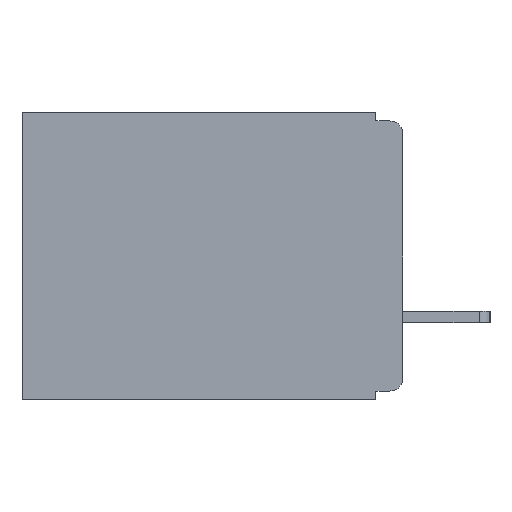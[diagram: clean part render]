
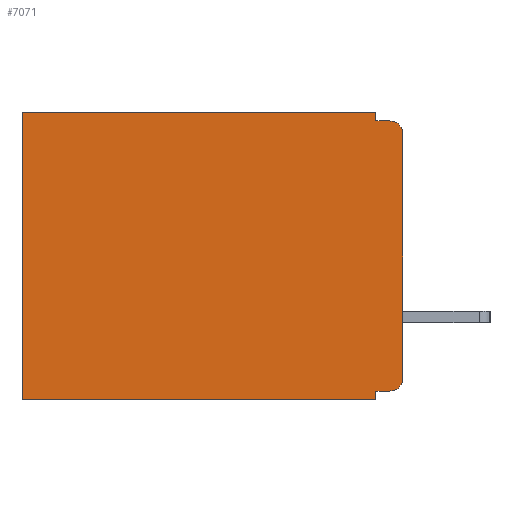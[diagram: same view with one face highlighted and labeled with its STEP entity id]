
A CAD part, left-side view. The second image highlights one B-rep face of the part: STEP entity #7071.
In plain terms, the highlighted planar face has unit normal (-1, 0, 0).
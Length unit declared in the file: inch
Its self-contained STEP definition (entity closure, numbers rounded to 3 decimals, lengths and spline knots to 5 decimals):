
#263 = DIRECTION ( 'NONE',  ( 0., 0., -1. ) ) ;
#1427 = EDGE_CURVE ( 'NONE', #22461, #13927, #12669, .T. ) ;
#1636 = CARTESIAN_POINT ( 'NONE',  ( 0.3, 0., -0.305 ) ) ;
#1752 = CARTESIAN_POINT ( 'NONE',  ( 0.3, 0., -0.01 ) ) ;
#1846 = CIRCLE ( 'NONE', #20642, 0.015 ) ;
#2323 = EDGE_CURVE ( 'NONE', #16897, #26285, #1846, .T. ) ;
#2445 = PLANE ( 'NONE',  #14420 ) ;
#2568 = LINE ( 'NONE', #6167, #17418 ) ;
#2995 = CARTESIAN_POINT ( 'NONE',  ( 0.3, 0.031, 0. ) ) ;
#4629 = CARTESIAN_POINT ( 'NONE',  ( 0.3, 0.031, -0.33 ) ) ;
#4655 = DIRECTION ( 'NONE',  ( 1., 0., 0. ) ) ;
#4882 = ORIENTED_EDGE ( 'NONE', *, *, #13076, .F. ) ;
#5349 = DIRECTION ( 'NONE',  ( 0., -1., 0. ) ) ;
#5453 = CARTESIAN_POINT ( 'NONE',  ( 0.3, 0.437, 0. ) ) ;
#5562 = ORIENTED_EDGE ( 'NONE', *, *, #15362, .F. ) ;
#5638 = ORIENTED_EDGE ( 'NONE', *, *, #25795, .F. ) ;
#5671 = EDGE_CURVE ( 'NONE', #23626, #6668, #13593, .T. ) ;
#5767 = VERTEX_POINT ( 'NONE', #4629 ) ;
#5918 = EDGE_CURVE ( 'NONE', #24119, #22461, #17615, .T. ) ;
#6129 = ORIENTED_EDGE ( 'NONE', *, *, #2323, .T. ) ;
#6167 = CARTESIAN_POINT ( 'NONE',  ( 0.3, 0., 0. ) ) ;
#6527 = LINE ( 'NONE', #26461, #23247 ) ;
#6556 = ORIENTED_EDGE ( 'NONE', *, *, #19718, .F. ) ;
#6668 = VERTEX_POINT ( 'NONE', #25015 ) ;
#7071 = ADVANCED_FACE ( 'NONE', ( #24930 ), #2445, .F. ) ;
#7114 = CIRCLE ( 'NONE', #18214, 0.015 ) ;
#9069 = DIRECTION ( 'NONE',  ( -1., 0., 0. ) ) ;
#9681 = ORIENTED_EDGE ( 'NONE', *, *, #21355, .T. ) ;
#10039 = VERTEX_POINT ( 'NONE', #13477 ) ;
#10430 = CARTESIAN_POINT ( 'NONE',  ( 0.3, 0., -0.32 ) ) ;
#10809 = VECTOR ( 'NONE', #22095, 39.37008 ) ;
#11043 = CARTESIAN_POINT ( 'NONE',  ( 0.3, 0., -0.33 ) ) ;
#11328 = CARTESIAN_POINT ( 'NONE',  ( 0.3, 0., -0.33 ) ) ;
#11842 = VECTOR ( 'NONE', #20567, 39.37008 ) ;
#11960 = VECTOR ( 'NONE', #5349, 39.37008 ) ;
#12669 = LINE ( 'NONE', #1752, #11960 ) ;
#13076 = EDGE_CURVE ( 'NONE', #10039, #5767, #15922, .T. ) ;
#13277 = DIRECTION ( 'NONE',  ( 0., 1., 0. ) ) ;
#13327 = VERTEX_POINT ( 'NONE', #18680 ) ;
#13381 = CARTESIAN_POINT ( 'NONE',  ( 0.3, 0.031, -0.01 ) ) ;
#13477 = CARTESIAN_POINT ( 'NONE',  ( 0.3, 0.031, -0.32 ) ) ;
#13593 = LINE ( 'NONE', #15315, #25007 ) ;
#13927 = VERTEX_POINT ( 'NONE', #18648 ) ;
#14420 = AXIS2_PLACEMENT_3D ( 'NONE', #11328, #4655, #20041 ) ;
#14569 = LINE ( 'NONE', #11043, #20295 ) ;
#14839 = DIRECTION ( 'NONE',  ( 0., 1., 0. ) ) ;
#15315 = CARTESIAN_POINT ( 'NONE',  ( 0.3, 0.437, -0.33 ) ) ;
#15362 = EDGE_CURVE ( 'NONE', #16897, #10039, #17183, .T. ) ;
#15366 = ORIENTED_EDGE ( 'NONE', *, *, #21829, .T. ) ;
#15611 = CARTESIAN_POINT ( 'NONE',  ( 0.3, 0.031, -0.33 ) ) ;
#15922 = LINE ( 'NONE', #15611, #10809 ) ;
#16897 = VERTEX_POINT ( 'NONE', #22459 ) ;
#17170 = EDGE_LOOP ( 'NONE', ( #6556, #9681, #21881, #23329, #15366, #23208, #5638, #4882, #5562, #6129 ) ) ;
#17183 = LINE ( 'NONE', #10430, #27898 ) ;
#17418 = VECTOR ( 'NONE', #25778, 39.37008 ) ;
#17615 = LINE ( 'NONE', #2995, #11842 ) ;
#18214 = AXIS2_PLACEMENT_3D ( 'NONE', #22086, #9069, #24244 ) ;
#18648 = CARTESIAN_POINT ( 'NONE',  ( 0.3, 0.015, -0.01 ) ) ;
#18680 = CARTESIAN_POINT ( 'NONE',  ( 0.3, 0., -0.025 ) ) ;
#19718 = EDGE_CURVE ( 'NONE', #13327, #26285, #6527, .T. ) ;
#20041 = DIRECTION ( 'NONE',  ( 0., 0., -1. ) ) ;
#20295 = VECTOR ( 'NONE', #13277, 39.37008 ) ;
#20567 = DIRECTION ( 'NONE',  ( 0., 0., -1. ) ) ;
#20580 = DIRECTION ( 'NONE',  ( -1., 0., 0. ) ) ;
#20642 = AXIS2_PLACEMENT_3D ( 'NONE', #26998, #20580, #23226 ) ;
#21355 = EDGE_CURVE ( 'NONE', #13327, #13927, #7114, .T. ) ;
#21829 = EDGE_CURVE ( 'NONE', #24119, #23626, #2568, .T. ) ;
#21881 = ORIENTED_EDGE ( 'NONE', *, *, #1427, .F. ) ;
#22086 = CARTESIAN_POINT ( 'NONE',  ( 0.3, 0.015, -0.025 ) ) ;
#22095 = DIRECTION ( 'NONE',  ( 0., 0., -1. ) ) ;
#22459 = CARTESIAN_POINT ( 'NONE',  ( 0.3, 0.015, -0.32 ) ) ;
#22461 = VERTEX_POINT ( 'NONE', #13381 ) ;
#23208 = ORIENTED_EDGE ( 'NONE', *, *, #5671, .T. ) ;
#23226 = DIRECTION ( 'NONE',  ( 0., 0., -1. ) ) ;
#23247 = VECTOR ( 'NONE', #263, 39.37008 ) ;
#23329 = ORIENTED_EDGE ( 'NONE', *, *, #5918, .F. ) ;
#23626 = VERTEX_POINT ( 'NONE', #5453 ) ;
#24119 = VERTEX_POINT ( 'NONE', #27127 ) ;
#24244 = DIRECTION ( 'NONE',  ( 0., 0., -1. ) ) ;
#24930 = FACE_OUTER_BOUND ( 'NONE', #17170, .T. ) ;
#25007 = VECTOR ( 'NONE', #28138, 39.37008 ) ;
#25015 = CARTESIAN_POINT ( 'NONE',  ( 0.3, 0.437, -0.33 ) ) ;
#25778 = DIRECTION ( 'NONE',  ( 0., 1., 0. ) ) ;
#25795 = EDGE_CURVE ( 'NONE', #5767, #6668, #14569, .T. ) ;
#26285 = VERTEX_POINT ( 'NONE', #1636 ) ;
#26461 = CARTESIAN_POINT ( 'NONE',  ( 0.3, 0., -0.33 ) ) ;
#26998 = CARTESIAN_POINT ( 'NONE',  ( 0.3, 0.015, -0.305 ) ) ;
#27127 = CARTESIAN_POINT ( 'NONE',  ( 0.3, 0.031, 0. ) ) ;
#27898 = VECTOR ( 'NONE', #14839, 39.37008 ) ;
#28138 = DIRECTION ( 'NONE',  ( 0., 0., -1. ) ) ;
